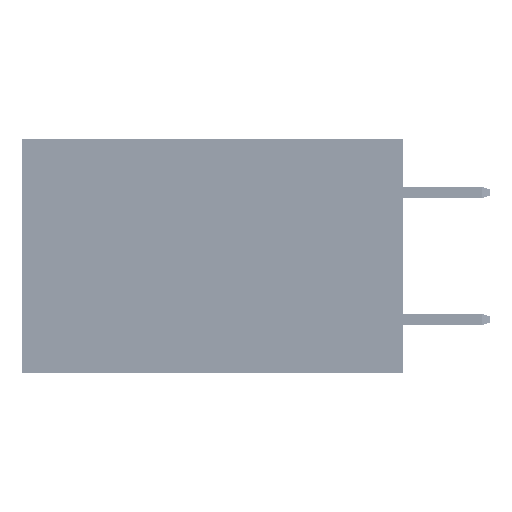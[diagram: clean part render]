
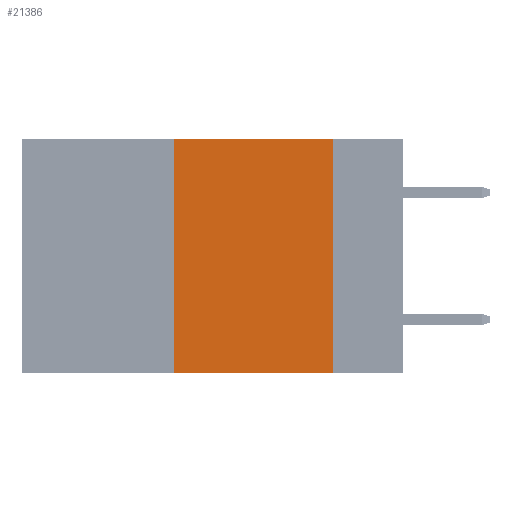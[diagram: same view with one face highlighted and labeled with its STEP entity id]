
A CAD part, left-side view. The second image highlights one B-rep face of the part: STEP entity #21386.
In plain terms, the highlighted planar face has unit normal (-1, 0, 0).
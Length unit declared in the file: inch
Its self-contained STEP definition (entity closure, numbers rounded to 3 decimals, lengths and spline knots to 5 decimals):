
#2239 = DIRECTION ( 'NONE',  ( 0., -1., 0. ) ) ;
#2356 = LINE ( 'NONE', #5725, #44615 ) ;
#3215 = FACE_OUTER_BOUND ( 'NONE', #4146, .T. ) ;
#4146 = EDGE_LOOP ( 'NONE', ( #6788, #26377, #33540, #43339 ) ) ;
#4737 = VERTEX_POINT ( 'NONE', #28996 ) ;
#5619 = VECTOR ( 'NONE', #40443, 39.37008 ) ;
#5725 = CARTESIAN_POINT ( 'NONE',  ( 0., 0.11, 0. ) ) ;
#6788 = ORIENTED_EDGE ( 'NONE', *, *, #15093, .F. ) ;
#8836 = CARTESIAN_POINT ( 'NONE',  ( 0., 0.36, 0. ) ) ;
#9410 = AXIS2_PLACEMENT_3D ( 'NONE', #21006, #32506, #36109 ) ;
#9769 = EDGE_CURVE ( 'NONE', #23538, #19141, #20379, .T. ) ;
#15093 = EDGE_CURVE ( 'NONE', #4737, #25327, #2356, .T. ) ;
#15574 = EDGE_CURVE ( 'NONE', #19141, #4737, #35138, .T. ) ;
#16937 = PLANE ( 'NONE',  #9410 ) ;
#19141 = VERTEX_POINT ( 'NONE', #27769 ) ;
#20379 = LINE ( 'NONE', #8836, #29057 ) ;
#21006 = CARTESIAN_POINT ( 'NONE',  ( 0., 0.6, 0. ) ) ;
#21386 = ADVANCED_FACE ( 'NONE', ( #3215 ), #16937, .F. ) ;
#21969 = CARTESIAN_POINT ( 'NONE',  ( 0., 0.6, -0.37 ) ) ;
#23538 = VERTEX_POINT ( 'NONE', #23797 ) ;
#23797 = CARTESIAN_POINT ( 'NONE',  ( 0., 0.36, -0.37 ) ) ;
#24027 = CARTESIAN_POINT ( 'NONE',  ( 0., 0.11, -0.37 ) ) ;
#25327 = VERTEX_POINT ( 'NONE', #24027 ) ;
#26051 = LINE ( 'NONE', #21969, #5619 ) ;
#26377 = ORIENTED_EDGE ( 'NONE', *, *, #15574, .F. ) ;
#27769 = CARTESIAN_POINT ( 'NONE',  ( 0., 0.36, 0. ) ) ;
#28996 = CARTESIAN_POINT ( 'NONE',  ( 0., 0.11, 0. ) ) ;
#29057 = VECTOR ( 'NONE', #34785, 39.37008 ) ;
#32506 = DIRECTION ( 'NONE',  ( 1., 0., 0. ) ) ;
#33540 = ORIENTED_EDGE ( 'NONE', *, *, #9769, .F. ) ;
#34785 = DIRECTION ( 'NONE',  ( 0., 0., 1. ) ) ;
#34900 = CARTESIAN_POINT ( 'NONE',  ( 0., 0.6, 0. ) ) ;
#35138 = LINE ( 'NONE', #34900, #45439 ) ;
#36109 = DIRECTION ( 'NONE',  ( 0., 0., -1. ) ) ;
#40443 = DIRECTION ( 'NONE',  ( 0., -1., 0. ) ) ;
#41571 = EDGE_CURVE ( 'NONE', #23538, #25327, #26051, .T. ) ;
#41754 = DIRECTION ( 'NONE',  ( 0., 0., -1. ) ) ;
#43339 = ORIENTED_EDGE ( 'NONE', *, *, #41571, .T. ) ;
#44615 = VECTOR ( 'NONE', #41754, 39.37008 ) ;
#45439 = VECTOR ( 'NONE', #2239, 39.37008 ) ;
